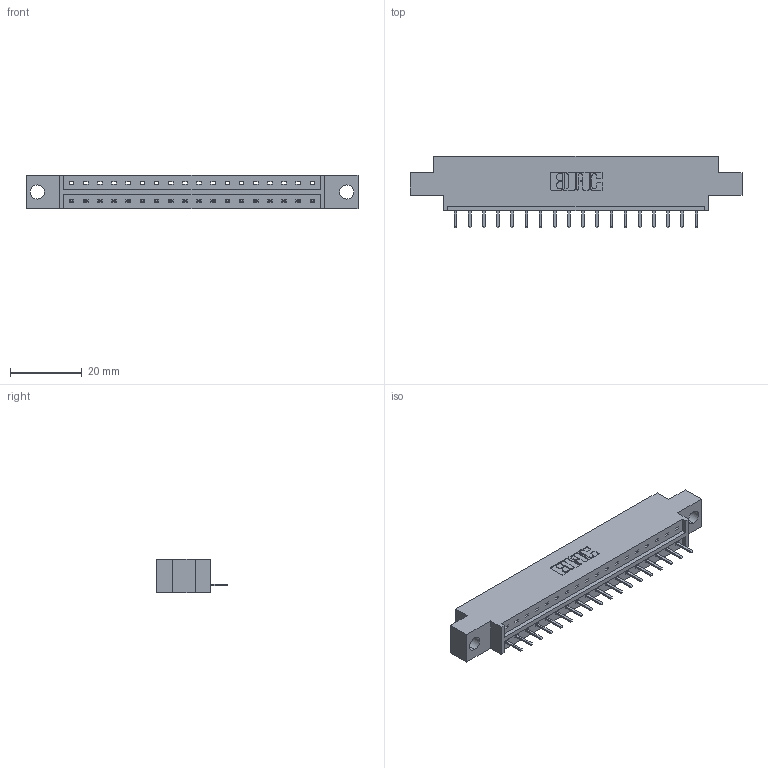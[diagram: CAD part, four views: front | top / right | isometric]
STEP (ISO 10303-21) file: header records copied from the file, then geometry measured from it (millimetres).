
FILE_DESCRIPTION (( 'STEP AP203' ), '1' );
FILE_NAME ('333-018-520-604.STEP', '2019-08-09T12:42:57', ( '' ), ( '' ), 'SwSTEP 2.0', 'SolidWorks 2016', '' );
FILE_SCHEMA (( 'CONFIG_CONTROL_DESIGN' ));
Length unit declared in the file: inch
Products named in the file (3): 333 Part_Offset - .156 Dia - TH; 333-018-520-604; 345-292-001_345-293-120
Assembly tree (19 placements, depth 2):
  333-018-520-604
    333 Part_Offset - .156 Dia - TH
    345-292-001_345-293-120  x18
Bounding box: 92.86 x 20.02 x 9.4 mm (x, y, z)
Volume: 8770.7 mm3; surface area: 9144.4 mm2
Topology: 19 solids, 19 shells, 1234 faces, 3635 edges, 2374 vertices
Faces by surface type: plane 866, cylinder 368
Entity records: 14357 total; most frequent: CARTESIAN_POINT 2500, ORIENTED_EDGE 2442, DIRECTION 2145, EDGE_CURVE 1221, VECTOR 1089, LINE 1089, VERTEX_POINT 810, AXIS2_PLACEMENT_3D 528
